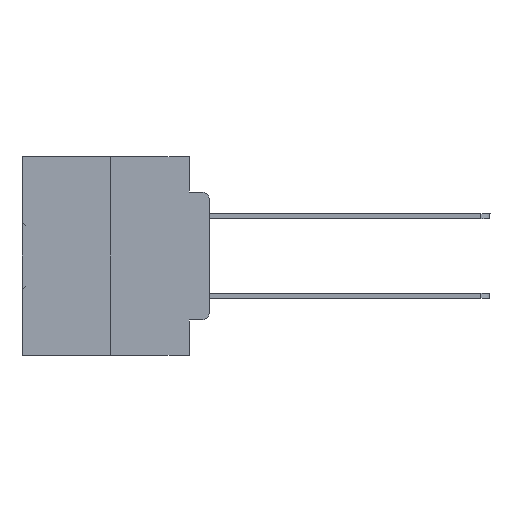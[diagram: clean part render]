
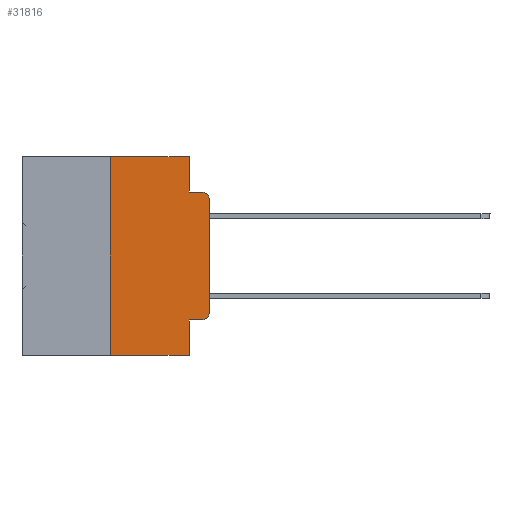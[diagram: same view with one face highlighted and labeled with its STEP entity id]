
A CAD part, left-side view. The second image highlights one B-rep face of the part: STEP entity #31816.
In plain terms, the highlighted planar face has unit normal (-1, 0, 0).
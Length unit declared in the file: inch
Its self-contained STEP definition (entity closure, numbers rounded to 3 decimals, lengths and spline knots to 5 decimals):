
#34 = ORIENTED_EDGE ( 'NONE', *, *, #27664, .F. ) ;
#311 = EDGE_CURVE ( 'NONE', #12964, #7666, #24041, .T. ) ;
#957 = CARTESIAN_POINT ( 'NONE',  ( 0., 0., 0. ) ) ;
#1614 = ORIENTED_EDGE ( 'NONE', *, *, #311, .T. ) ;
#1663 = CARTESIAN_POINT ( 'NONE',  ( 0., 0.473, 0. ) ) ;
#1784 = ORIENTED_EDGE ( 'NONE', *, *, #14441, .F. ) ;
#2388 = VERTEX_POINT ( 'NONE', #18657 ) ;
#2688 = DIRECTION ( 'NONE',  ( 0., -1., 0. ) ) ;
#4006 = CIRCLE ( 'NONE', #11106, 0.02 ) ;
#4047 = EDGE_CURVE ( 'NONE', #35112, #2388, #4006, .T. ) ;
#5151 = ORIENTED_EDGE ( 'NONE', *, *, #13146, .T. ) ;
#6258 = DIRECTION ( 'NONE',  ( 0., 0., -1. ) ) ;
#6746 = DIRECTION ( 'NONE',  ( 0., 0., -1. ) ) ;
#7151 = CARTESIAN_POINT ( 'NONE',  ( 0., 0.051, 0. ) ) ;
#7232 = VECTOR ( 'NONE', #20112, 39.37008 ) ;
#7666 = VERTEX_POINT ( 'NONE', #14277 ) ;
#8154 = EDGE_CURVE ( 'NONE', #35882, #7666, #19199, .T. ) ;
#8653 = EDGE_CURVE ( 'NONE', #11354, #35112, #14161, .T. ) ;
#9409 = DIRECTION ( 'NONE',  ( 0., 0., -1. ) ) ;
#9596 = ORIENTED_EDGE ( 'NONE', *, *, #8653, .T. ) ;
#9883 = CARTESIAN_POINT ( 'NONE',  ( 0., 0.473, 0. ) ) ;
#10183 = EDGE_CURVE ( 'NONE', #29239, #27588, #28000, .T. ) ;
#10273 = EDGE_LOOP ( 'NONE', ( #32547, #1614, #30646, #19162, #1784, #27049, #5151, #34, #9596, #32869 ) ) ;
#10531 = DIRECTION ( 'NONE',  ( 0., -1., 0. ) ) ;
#11106 = AXIS2_PLACEMENT_3D ( 'NONE', #28999, #14764, #6258 ) ;
#11354 = VERTEX_POINT ( 'NONE', #18299 ) ;
#12404 = LINE ( 'NONE', #1663, #13056 ) ;
#12576 = CARTESIAN_POINT ( 'NONE',  ( 0., 0.051, 0. ) ) ;
#12954 = DIRECTION ( 'NONE',  ( 0., -1., 0. ) ) ;
#12964 = VERTEX_POINT ( 'NONE', #23701 ) ;
#12967 = VECTOR ( 'NONE', #10531, 39.37008 ) ;
#13056 = VECTOR ( 'NONE', #12954, 39.37008 ) ;
#13146 = EDGE_CURVE ( 'NONE', #29239, #24899, #35893, .T. ) ;
#13255 = VECTOR ( 'NONE', #2688, 39.37008 ) ;
#14161 = LINE ( 'NONE', #16959, #7232 ) ;
#14277 = CARTESIAN_POINT ( 'NONE',  ( 0., 0.02, -0.0885 ) ) ;
#14441 = EDGE_CURVE ( 'NONE', #27588, #31312, #12404, .T. ) ;
#14764 = DIRECTION ( 'NONE',  ( -1., 0., 0. ) ) ;
#15343 = LINE ( 'NONE', #24207, #35764 ) ;
#15503 = AXIS2_PLACEMENT_3D ( 'NONE', #9883, #15800, #6746 ) ;
#15800 = DIRECTION ( 'NONE',  ( 1., 0., 0. ) ) ;
#16959 = CARTESIAN_POINT ( 'NONE',  ( 0., 0.051, -0.4115 ) ) ;
#17025 = CARTESIAN_POINT ( 'NONE',  ( 0., 0.25, 0. ) ) ;
#18299 = CARTESIAN_POINT ( 'NONE',  ( 0., 0.051, -0.4115 ) ) ;
#18657 = CARTESIAN_POINT ( 'NONE',  ( 0., 0., -0.3915 ) ) ;
#19016 = CARTESIAN_POINT ( 'NONE',  ( 0., 0.051, -0.0885 ) ) ;
#19162 = ORIENTED_EDGE ( 'NONE', *, *, #30974, .F. ) ;
#19164 = DIRECTION ( 'NONE',  ( 0., 0., 1. ) ) ;
#19199 = LINE ( 'NONE', #19016, #13255 ) ;
#20112 = DIRECTION ( 'NONE',  ( 0., -1., 0. ) ) ;
#20558 = CARTESIAN_POINT ( 'NONE',  ( 0., 0.02, -0.1085 ) ) ;
#20593 = CARTESIAN_POINT ( 'NONE',  ( 0., 0.051, -0.5 ) ) ;
#20862 = CARTESIAN_POINT ( 'NONE',  ( 0., 0.051, -0.0885 ) ) ;
#21181 = PLANE ( 'NONE',  #15503 ) ;
#21663 = VECTOR ( 'NONE', #19164, 39.37008 ) ;
#22047 = CARTESIAN_POINT ( 'NONE',  ( 0., 0.473, -0.5 ) ) ;
#23701 = CARTESIAN_POINT ( 'NONE',  ( 0., 0., -0.1085 ) ) ;
#24041 = CIRCLE ( 'NONE', #34686, 0.02 ) ;
#24207 = CARTESIAN_POINT ( 'NONE',  ( 0., 0.051, 0. ) ) ;
#24488 = CARTESIAN_POINT ( 'NONE',  ( 0., 0.02, -0.4115 ) ) ;
#24801 = EDGE_CURVE ( 'NONE', #2388, #12964, #34070, .T. ) ;
#24899 = VERTEX_POINT ( 'NONE', #20593 ) ;
#26444 = LINE ( 'NONE', #12576, #32001 ) ;
#27049 = ORIENTED_EDGE ( 'NONE', *, *, #10183, .F. ) ;
#27391 = CARTESIAN_POINT ( 'NONE',  ( 0., 0.25, -0.5 ) ) ;
#27588 = VERTEX_POINT ( 'NONE', #17025 ) ;
#27664 = EDGE_CURVE ( 'NONE', #11354, #24899, #15343, .T. ) ;
#28000 = LINE ( 'NONE', #30588, #21663 ) ;
#28524 = DIRECTION ( 'NONE',  ( 0., 0., 1. ) ) ;
#28577 = VECTOR ( 'NONE', #28524, 39.37008 ) ;
#28999 = CARTESIAN_POINT ( 'NONE',  ( 0., 0.02, -0.3915 ) ) ;
#29239 = VERTEX_POINT ( 'NONE', #27391 ) ;
#30588 = CARTESIAN_POINT ( 'NONE',  ( 0., 0.25, 0. ) ) ;
#30646 = ORIENTED_EDGE ( 'NONE', *, *, #8154, .F. ) ;
#30974 = EDGE_CURVE ( 'NONE', #31312, #35882, #26444, .T. ) ;
#31312 = VERTEX_POINT ( 'NONE', #7151 ) ;
#31816 = ADVANCED_FACE ( 'NONE', ( #31905 ), #21181, .F. ) ;
#31905 = FACE_OUTER_BOUND ( 'NONE', #10273, .T. ) ;
#32001 = VECTOR ( 'NONE', #35146, 39.37008 ) ;
#32186 = DIRECTION ( 'NONE',  ( 0., 0., -1. ) ) ;
#32547 = ORIENTED_EDGE ( 'NONE', *, *, #24801, .T. ) ;
#32869 = ORIENTED_EDGE ( 'NONE', *, *, #4047, .T. ) ;
#34070 = LINE ( 'NONE', #957, #28577 ) ;
#34598 = DIRECTION ( 'NONE',  ( -1., 0., 0. ) ) ;
#34686 = AXIS2_PLACEMENT_3D ( 'NONE', #20558, #34598, #32186 ) ;
#35112 = VERTEX_POINT ( 'NONE', #24488 ) ;
#35146 = DIRECTION ( 'NONE',  ( 0., 0., -1. ) ) ;
#35764 = VECTOR ( 'NONE', #9409, 39.37008 ) ;
#35882 = VERTEX_POINT ( 'NONE', #20862 ) ;
#35893 = LINE ( 'NONE', #22047, #12967 ) ;
